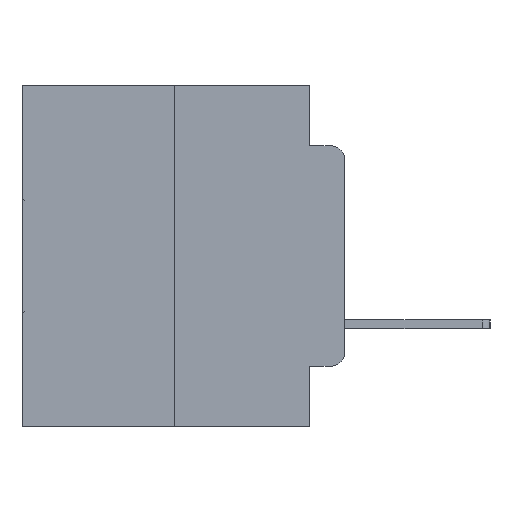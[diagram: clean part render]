
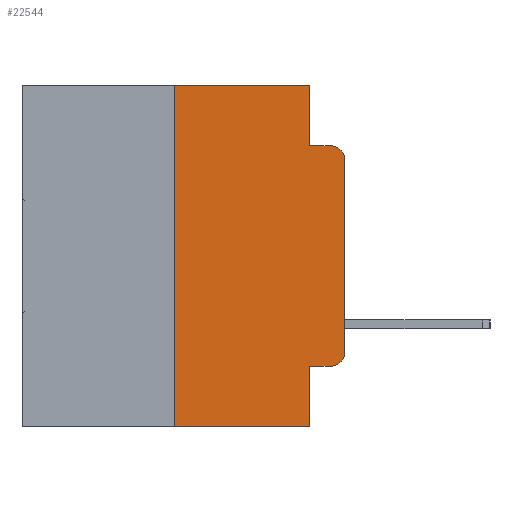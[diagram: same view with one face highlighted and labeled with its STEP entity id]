
A CAD part, left-side view. The second image highlights one B-rep face of the part: STEP entity #22544.
In plain terms, the highlighted planar face has unit normal (-1, 0, 0).
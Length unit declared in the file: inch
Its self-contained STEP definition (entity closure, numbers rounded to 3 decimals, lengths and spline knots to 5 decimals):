
#806 = CARTESIAN_POINT ( 'NONE',  ( 0., 0.473, -0.5 ) ) ;
#867 = CARTESIAN_POINT ( 'NONE',  ( 0., 0., -0.3915 ) ) ;
#924 = CARTESIAN_POINT ( 'NONE',  ( 0., 0.25, 0. ) ) ;
#996 = VECTOR ( 'NONE', #16494, 39.37008 ) ;
#1576 = ORIENTED_EDGE ( 'NONE', *, *, #23651, .F. ) ;
#1637 = DIRECTION ( 'NONE',  ( 0., -1., 0. ) ) ;
#1818 = DIRECTION ( 'NONE',  ( 0., 0., -1. ) ) ;
#2105 = EDGE_CURVE ( 'NONE', #7918, #9646, #11005, .T. ) ;
#2215 = DIRECTION ( 'NONE',  ( 0., -1., 0. ) ) ;
#2310 = ORIENTED_EDGE ( 'NONE', *, *, #2105, .F. ) ;
#2672 = VECTOR ( 'NONE', #14229, 39.37008 ) ;
#4422 = DIRECTION ( 'NONE',  ( 0., 0., -1. ) ) ;
#4517 = DIRECTION ( 'NONE',  ( 0., 0., 1. ) ) ;
#4545 = VERTEX_POINT ( 'NONE', #10431 ) ;
#5012 = CARTESIAN_POINT ( 'NONE',  ( 0., 0.051, -0.5 ) ) ;
#5352 = CARTESIAN_POINT ( 'NONE',  ( 0., 0.051, 0. ) ) ;
#5510 = EDGE_CURVE ( 'NONE', #4545, #19672, #27239, .T. ) ;
#5564 = EDGE_CURVE ( 'NONE', #6639, #20733, #13701, .T. ) ;
#5723 = CARTESIAN_POINT ( 'NONE',  ( 0., 0.02, -0.0885 ) ) ;
#5854 = VECTOR ( 'NONE', #1637, 39.37008 ) ;
#6211 = FACE_OUTER_BOUND ( 'NONE', #7888, .T. ) ;
#6639 = VERTEX_POINT ( 'NONE', #8651 ) ;
#6918 = VECTOR ( 'NONE', #4517, 39.37008 ) ;
#7046 = VERTEX_POINT ( 'NONE', #19314 ) ;
#7171 = LINE ( 'NONE', #25482, #996 ) ;
#7888 = EDGE_LOOP ( 'NONE', ( #9220, #10635, #1576, #2310, #28745, #14982, #10283, #20089, #22930, #23293 ) ) ;
#7918 = VERTEX_POINT ( 'NONE', #5352 ) ;
#8482 = VERTEX_POINT ( 'NONE', #5012 ) ;
#8498 = DIRECTION ( 'NONE',  ( -1., 0., 0. ) ) ;
#8570 = AXIS2_PLACEMENT_3D ( 'NONE', #22729, #18242, #4422 ) ;
#8651 = CARTESIAN_POINT ( 'NONE',  ( 0., 0.02, -0.4115 ) ) ;
#9022 = EDGE_CURVE ( 'NONE', #22904, #7918, #17510, .T. ) ;
#9220 = ORIENTED_EDGE ( 'NONE', *, *, #11958, .T. ) ;
#9398 = CARTESIAN_POINT ( 'NONE',  ( 0., 0.051, 0. ) ) ;
#9646 = VERTEX_POINT ( 'NONE', #18548 ) ;
#10283 = ORIENTED_EDGE ( 'NONE', *, *, #27688, .T. ) ;
#10431 = CARTESIAN_POINT ( 'NONE',  ( 0., 0., -0.1085 ) ) ;
#10635 = ORIENTED_EDGE ( 'NONE', *, *, #5510, .T. ) ;
#11005 = LINE ( 'NONE', #15236, #22553 ) ;
#11243 = PLANE ( 'NONE',  #8570 ) ;
#11818 = LINE ( 'NONE', #9398, #28515 ) ;
#11958 = EDGE_CURVE ( 'NONE', #20733, #4545, #20352, .T. ) ;
#13701 = CIRCLE ( 'NONE', #24639, 0.02 ) ;
#14229 = DIRECTION ( 'NONE',  ( 0., 0., 1. ) ) ;
#14982 = ORIENTED_EDGE ( 'NONE', *, *, #29482, .F. ) ;
#15236 = CARTESIAN_POINT ( 'NONE',  ( 0., 0.051, 0. ) ) ;
#15684 = DIRECTION ( 'NONE',  ( -1., 0., 0. ) ) ;
#16494 = DIRECTION ( 'NONE',  ( 0., -1., 0. ) ) ;
#17008 = DIRECTION ( 'NONE',  ( 0., -1., 0. ) ) ;
#17052 = AXIS2_PLACEMENT_3D ( 'NONE', #22292, #8498, #24509 ) ;
#17117 = LINE ( 'NONE', #806, #23856 ) ;
#17510 = LINE ( 'NONE', #29532, #28758 ) ;
#18242 = DIRECTION ( 'NONE',  ( 1., 0., 0. ) ) ;
#18411 = EDGE_CURVE ( 'NONE', #21526, #8482, #11818, .T. ) ;
#18548 = CARTESIAN_POINT ( 'NONE',  ( 0., 0.051, -0.0885 ) ) ;
#18578 = DIRECTION ( 'NONE',  ( 0., 0., -1. ) ) ;
#19314 = CARTESIAN_POINT ( 'NONE',  ( 0., 0.25, -0.5 ) ) ;
#19672 = VERTEX_POINT ( 'NONE', #5723 ) ;
#19909 = LINE ( 'NONE', #22902, #6918 ) ;
#20089 = ORIENTED_EDGE ( 'NONE', *, *, #18411, .F. ) ;
#20117 = CARTESIAN_POINT ( 'NONE',  ( 0., 0.051, -0.0885 ) ) ;
#20352 = LINE ( 'NONE', #27814, #2672 ) ;
#20733 = VERTEX_POINT ( 'NONE', #867 ) ;
#21526 = VERTEX_POINT ( 'NONE', #28895 ) ;
#22292 = CARTESIAN_POINT ( 'NONE',  ( 0., 0.02, -0.1085 ) ) ;
#22544 = ADVANCED_FACE ( 'NONE', ( #6211 ), #11243, .F. ) ;
#22553 = VECTOR ( 'NONE', #28750, 39.37008 ) ;
#22729 = CARTESIAN_POINT ( 'NONE',  ( 0., 0.473, 0. ) ) ;
#22902 = CARTESIAN_POINT ( 'NONE',  ( 0., 0.25, 0. ) ) ;
#22904 = VERTEX_POINT ( 'NONE', #924 ) ;
#22930 = ORIENTED_EDGE ( 'NONE', *, *, #25274, .T. ) ;
#23293 = ORIENTED_EDGE ( 'NONE', *, *, #5564, .T. ) ;
#23447 = LINE ( 'NONE', #20117, #5854 ) ;
#23651 = EDGE_CURVE ( 'NONE', #9646, #19672, #23447, .T. ) ;
#23856 = VECTOR ( 'NONE', #17008, 39.37008 ) ;
#24509 = DIRECTION ( 'NONE',  ( 0., 0., -1. ) ) ;
#24639 = AXIS2_PLACEMENT_3D ( 'NONE', #29166, #15684, #1818 ) ;
#25274 = EDGE_CURVE ( 'NONE', #21526, #6639, #7171, .T. ) ;
#25482 = CARTESIAN_POINT ( 'NONE',  ( 0., 0.051, -0.4115 ) ) ;
#27239 = CIRCLE ( 'NONE', #17052, 0.02 ) ;
#27688 = EDGE_CURVE ( 'NONE', #7046, #8482, #17117, .T. ) ;
#27814 = CARTESIAN_POINT ( 'NONE',  ( 0., 0., 0. ) ) ;
#28515 = VECTOR ( 'NONE', #18578, 39.37008 ) ;
#28745 = ORIENTED_EDGE ( 'NONE', *, *, #9022, .F. ) ;
#28750 = DIRECTION ( 'NONE',  ( 0., 0., -1. ) ) ;
#28758 = VECTOR ( 'NONE', #2215, 39.37008 ) ;
#28895 = CARTESIAN_POINT ( 'NONE',  ( 0., 0.051, -0.4115 ) ) ;
#29166 = CARTESIAN_POINT ( 'NONE',  ( 0., 0.02, -0.3915 ) ) ;
#29482 = EDGE_CURVE ( 'NONE', #7046, #22904, #19909, .T. ) ;
#29532 = CARTESIAN_POINT ( 'NONE',  ( 0., 0.473, 0. ) ) ;
